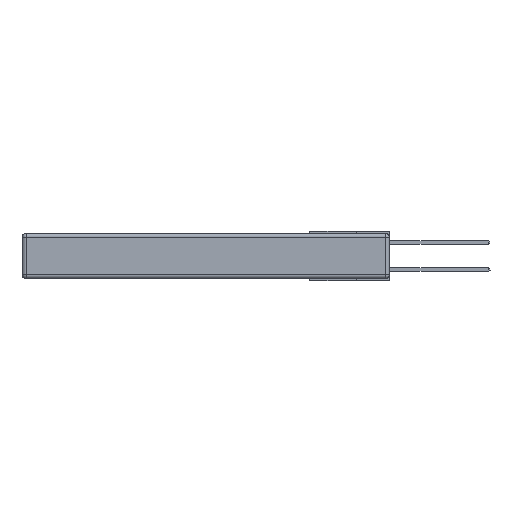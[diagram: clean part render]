
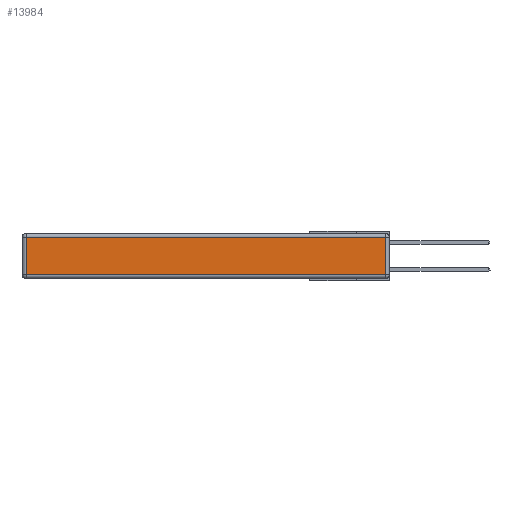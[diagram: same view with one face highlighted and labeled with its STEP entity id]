
A CAD part, left-side view. The second image highlights one B-rep face of the part: STEP entity #13984.
In plain terms, the highlighted planar face has unit normal (-1, 0, 0).
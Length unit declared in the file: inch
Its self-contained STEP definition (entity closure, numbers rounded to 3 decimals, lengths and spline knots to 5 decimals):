
#592 = EDGE_CURVE ( 'NONE', #21048, #21027, #9190, .T. ) ;
#819 = EDGE_CURVE ( 'NONE', #21027, #22130, #5326, .T. ) ;
#1693 = LINE ( 'NONE', #9518, #13143 ) ;
#2006 = DIRECTION ( 'NONE',  ( 0., -1., 0. ) ) ;
#2640 = ORIENTED_EDGE ( 'NONE', *, *, #22723, .T. ) ;
#3213 = LINE ( 'NONE', #5718, #5239 ) ;
#3561 = ORIENTED_EDGE ( 'NONE', *, *, #8207, .T. ) ;
#3877 = CARTESIAN_POINT ( 'NONE',  ( 0., 0., -0.313 ) ) ;
#4750 = CARTESIAN_POINT ( 'NONE',  ( 0., 2.72, -0.313 ) ) ;
#5107 = CARTESIAN_POINT ( 'NONE',  ( 0., 2.72, -0.343 ) ) ;
#5239 = VECTOR ( 'NONE', #7459, 39.37008 ) ;
#5326 = LINE ( 'NONE', #3877, #24224 ) ;
#5718 = CARTESIAN_POINT ( 'NONE',  ( 0., 2.75, -0.03 ) ) ;
#7405 = VECTOR ( 'NONE', #19954, 39.37008 ) ;
#7459 = DIRECTION ( 'NONE',  ( 0., 1., 0. ) ) ;
#7769 = AXIS2_PLACEMENT_3D ( 'NONE', #8251, #14018, #21452 ) ;
#8207 = EDGE_CURVE ( 'NONE', #22130, #18258, #1693, .T. ) ;
#8251 = CARTESIAN_POINT ( 'NONE',  ( 0., 0., -0.343 ) ) ;
#9190 = LINE ( 'NONE', #5107, #7405 ) ;
#9518 = CARTESIAN_POINT ( 'NONE',  ( 0., 0.03, -0.343 ) ) ;
#9789 = CARTESIAN_POINT ( 'NONE',  ( 0., 0.03, -0.313 ) ) ;
#10109 = CARTESIAN_POINT ( 'NONE',  ( 0., 0.03, -0.03 ) ) ;
#11968 = PLANE ( 'NONE',  #7769 ) ;
#13143 = VECTOR ( 'NONE', #15217, 39.37008 ) ;
#13984 = ADVANCED_FACE ( 'NONE', ( #20230 ), #11968, .T. ) ;
#14018 = DIRECTION ( 'NONE',  ( -1., 0., 0. ) ) ;
#15217 = DIRECTION ( 'NONE',  ( 0., 0., 1. ) ) ;
#16128 = ORIENTED_EDGE ( 'NONE', *, *, #819, .T. ) ;
#16143 = EDGE_LOOP ( 'NONE', ( #16128, #3561, #2640, #20730 ) ) ;
#16211 = CARTESIAN_POINT ( 'NONE',  ( 0., 2.72, -0.03 ) ) ;
#18258 = VERTEX_POINT ( 'NONE', #10109 ) ;
#19954 = DIRECTION ( 'NONE',  ( 0., 0., -1. ) ) ;
#20230 = FACE_OUTER_BOUND ( 'NONE', #16143, .T. ) ;
#20730 = ORIENTED_EDGE ( 'NONE', *, *, #592, .T. ) ;
#21027 = VERTEX_POINT ( 'NONE', #4750 ) ;
#21048 = VERTEX_POINT ( 'NONE', #16211 ) ;
#21452 = DIRECTION ( 'NONE',  ( 0., 0., 1. ) ) ;
#22130 = VERTEX_POINT ( 'NONE', #9789 ) ;
#22723 = EDGE_CURVE ( 'NONE', #18258, #21048, #3213, .T. ) ;
#24224 = VECTOR ( 'NONE', #2006, 39.37008 ) ;
